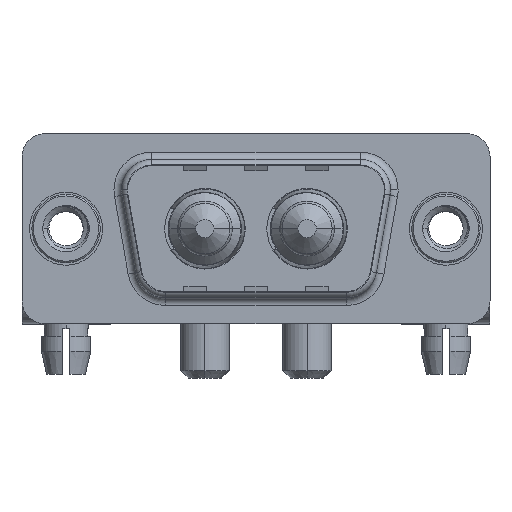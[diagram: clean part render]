
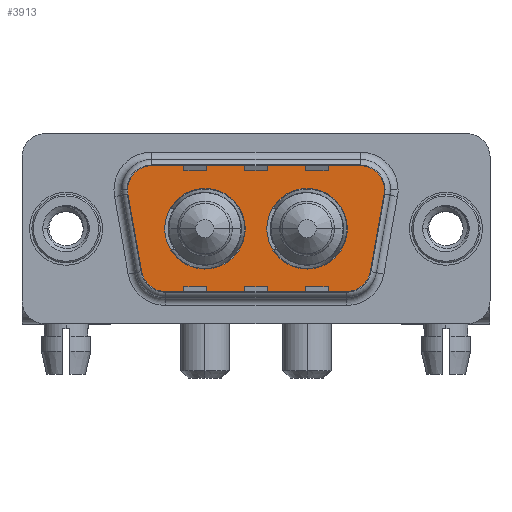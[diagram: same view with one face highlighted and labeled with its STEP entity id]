
A CAD part, top view. The second image highlights one B-rep face of the part: STEP entity #3913.
In plain terms, the highlighted planar face has unit normal (0, 0, 1).
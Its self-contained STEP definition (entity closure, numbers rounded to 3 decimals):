
#219 = ORIENTED_EDGE ( 'NONE', *, *, #4548, .T. ) ;
#256 = DIRECTION ( 'NONE',  ( -1., 0., 0. ) ) ;
#280 = CIRCLE ( 'NONE', #12714, 2.65 ) ;
#438 = VERTEX_POINT ( 'NONE', #11840 ) ;
#508 = VERTEX_POINT ( 'NONE', #8489 ) ;
#543 = CARTESIAN_POINT ( 'NONE',  ( 9.14, 0., 0. ) ) ;
#620 = AXIS2_PLACEMENT_3D ( 'NONE', #3584, #2506, #8239 ) ;
#798 = ORIENTED_EDGE ( 'NONE', *, *, #2090, .T. ) ;
#818 = EDGE_CURVE ( 'NONE', #6148, #5850, #7946, .T. ) ;
#905 = CARTESIAN_POINT ( 'NONE',  ( 4.489, -3.247, 0. ) ) ;
#919 = DIRECTION ( 'NONE',  ( 0., 0., 1. ) ) ;
#965 = CARTESIAN_POINT ( 'NONE',  ( 6.459, -4.9, 0. ) ) ;
#978 = EDGE_CURVE ( 'NONE', #4302, #438, #5430, .T. ) ;
#1011 = ORIENTED_EDGE ( 'NONE', *, *, #11360, .T. ) ;
#1084 = ORIENTED_EDGE ( 'NONE', *, *, #3416, .F. ) ;
#1127 = DIRECTION ( 'NONE',  ( 0., 0., 1. ) ) ;
#1158 = ORIENTED_EDGE ( 'NONE', *, *, #5422, .T. ) ;
#1280 = VECTOR ( 'NONE', #6122, 1000. ) ;
#1471 = ORIENTED_EDGE ( 'NONE', *, *, #11089, .F. ) ;
#1512 = DIRECTION ( 'NONE',  ( -1., 0., 0. ) ) ;
#1621 = CARTESIAN_POINT ( 'NONE',  ( 21.564, 2.9, 0. ) ) ;
#1681 = VERTEX_POINT ( 'NONE', #15098 ) ;
#2090 = EDGE_CURVE ( 'NONE', #1681, #9405, #5694, .T. ) ;
#2286 = AXIS2_PLACEMENT_3D ( 'NONE', #11740, #12900, #14204 ) ;
#2357 = VERTEX_POINT ( 'NONE', #6138 ) ;
#2362 = DIRECTION ( 'NONE',  ( 1., 0., 0. ) ) ;
#2506 = DIRECTION ( 'NONE',  ( 0., 0., 1. ) ) ;
#2527 = AXIS2_PLACEMENT_3D ( 'NONE', #4355, #4288, #8854 ) ;
#2708 = EDGE_CURVE ( 'NONE', #3065, #6148, #3999, .T. ) ;
#3010 = CIRCLE ( 'NONE', #2527, 2. ) ;
#3065 = VERTEX_POINT ( 'NONE', #10434 ) ;
#3349 = ORIENTED_EDGE ( 'NONE', *, *, #2708, .T. ) ;
#3353 = DIRECTION ( 'NONE',  ( 0.174, -0.985, 0. ) ) ;
#3416 = EDGE_CURVE ( 'NONE', #10693, #4105, #11099, .T. ) ;
#3494 = DIRECTION ( 'NONE',  ( -1., 0., 0. ) ) ;
#3502 = DIRECTION ( 'NONE',  ( 0., 0., 1. ) ) ;
#3505 = EDGE_CURVE ( 'NONE', #508, #3065, #12966, .T. ) ;
#3518 = AXIS2_PLACEMENT_3D ( 'NONE', #5768, #14240, #256 ) ;
#3584 = CARTESIAN_POINT ( 'NONE',  ( 9.14, 0., 0. ) ) ;
#3783 = AXIS2_PLACEMENT_3D ( 'NONE', #9064, #11437, #12652 ) ;
#3913 = ADVANCED_FACE ( 'NONE', ( #11501, #7924, #6779 ), #11579, .T. ) ;
#3999 = CIRCLE ( 'NONE', #2286, 2. ) ;
#4105 = VERTEX_POINT ( 'NONE', #12807 ) ;
#4218 = ORIENTED_EDGE ( 'NONE', *, *, #978, .F. ) ;
#4288 = DIRECTION ( 'NONE',  ( 0., 0., 1. ) ) ;
#4302 = VERTEX_POINT ( 'NONE', #8522 ) ;
#4355 = CARTESIAN_POINT ( 'NONE',  ( 18.541, -2.9, 0. ) ) ;
#4548 = EDGE_CURVE ( 'NONE', #13067, #508, #13030, .T. ) ;
#4737 = CARTESIAN_POINT ( 'NONE',  ( 5.436, 4.9, 0. ) ) ;
#4970 = DIRECTION ( 'NONE',  ( 1., 0., 0. ) ) ;
#5217 = LINE ( 'NONE', #9941, #1280 ) ;
#5422 = EDGE_CURVE ( 'NONE', #5850, #1681, #10359, .T. ) ;
#5430 = CIRCLE ( 'NONE', #14442, 2.65 ) ;
#5577 = CARTESIAN_POINT ( 'NONE',  ( 19.564, 2.9, 0. ) ) ;
#5694 = LINE ( 'NONE', #965, #8126 ) ;
#5768 = CARTESIAN_POINT ( 'NONE',  ( 19.564, 2.9, 0. ) ) ;
#5775 = CARTESIAN_POINT ( 'NONE',  ( 3.466, 2.553, 0. ) ) ;
#5850 = VERTEX_POINT ( 'NONE', #905 ) ;
#6122 = DIRECTION ( 'NONE',  ( 0.174, 0.985, 0. ) ) ;
#6138 = CARTESIAN_POINT ( 'NONE',  ( 21.534, 2.553, 0. ) ) ;
#6148 = VERTEX_POINT ( 'NONE', #5775 ) ;
#6239 = CIRCLE ( 'NONE', #12806, 2. ) ;
#6385 = AXIS2_PLACEMENT_3D ( 'NONE', #543, #8714, #4970 ) ;
#6779 = FACE_OUTER_BOUND ( 'NONE', #10398, .T. ) ;
#6901 = CARTESIAN_POINT ( 'NONE',  ( 20.511, -3.247, 0. ) ) ;
#7263 = VERTEX_POINT ( 'NONE', #6901 ) ;
#7321 = CARTESIAN_POINT ( 'NONE',  ( 15.86, 0., 0. ) ) ;
#7867 = CARTESIAN_POINT ( 'NONE',  ( 18.541, -4.9, 0. ) ) ;
#7924 = FACE_BOUND ( 'NONE', #9771, .T. ) ;
#7946 = LINE ( 'NONE', #8953, #8824 ) ;
#8126 = VECTOR ( 'NONE', #13867, 1000. ) ;
#8239 = DIRECTION ( 'NONE',  ( 1., 0., 0. ) ) ;
#8489 = CARTESIAN_POINT ( 'NONE',  ( 19.564, 4.9, 0. ) ) ;
#8522 = CARTESIAN_POINT ( 'NONE',  ( 13.21, 0., 0. ) ) ;
#8529 = DIRECTION ( 'NONE',  ( 1., 0., 0. ) ) ;
#8714 = DIRECTION ( 'NONE',  ( 0., 0., 1. ) ) ;
#8824 = VECTOR ( 'NONE', #3353, 1000. ) ;
#8844 = ORIENTED_EDGE ( 'NONE', *, *, #11159, .F. ) ;
#8854 = DIRECTION ( 'NONE',  ( 1., 0., 0. ) ) ;
#8953 = CARTESIAN_POINT ( 'NONE',  ( 3.466, 2.553, 0. ) ) ;
#9000 = CARTESIAN_POINT ( 'NONE',  ( 18.541, -2.9, 0. ) ) ;
#9013 = ORIENTED_EDGE ( 'NONE', *, *, #3505, .T. ) ;
#9064 = CARTESIAN_POINT ( 'NONE',  ( 6.459, -2.9, 0. ) ) ;
#9405 = VERTEX_POINT ( 'NONE', #7867 ) ;
#9673 = DIRECTION ( 'NONE',  ( 0., 0., 1. ) ) ;
#9771 = EDGE_LOOP ( 'NONE', ( #8844, #1084 ) ) ;
#9941 = CARTESIAN_POINT ( 'NONE',  ( 21.534, 2.553, 0. ) ) ;
#10254 = EDGE_CURVE ( 'NONE', #7263, #2357, #5217, .T. ) ;
#10359 = CIRCLE ( 'NONE', #3783, 2. ) ;
#10398 = EDGE_LOOP ( 'NONE', ( #1011, #12518, #14251, #219, #9013, #3349, #13445, #1158, #798 ) ) ;
#10434 = CARTESIAN_POINT ( 'NONE',  ( 5.436, 4.9, 0. ) ) ;
#10693 = VERTEX_POINT ( 'NONE', #12137 ) ;
#10813 = CARTESIAN_POINT ( 'NONE',  ( 15.86, 0., 0. ) ) ;
#11089 = EDGE_CURVE ( 'NONE', #438, #4302, #280, .T. ) ;
#11099 = CIRCLE ( 'NONE', #620, 2.65 ) ;
#11159 = EDGE_CURVE ( 'NONE', #4105, #10693, #13213, .T. ) ;
#11360 = EDGE_CURVE ( 'NONE', #9405, #7263, #3010, .T. ) ;
#11395 = EDGE_LOOP ( 'NONE', ( #1471, #4218 ) ) ;
#11436 = DIRECTION ( 'NONE',  ( 1., 0., 0. ) ) ;
#11437 = DIRECTION ( 'NONE',  ( 0., 0., 1. ) ) ;
#11501 = FACE_BOUND ( 'NONE', #11395, .T. ) ;
#11579 = PLANE ( 'NONE',  #14972 ) ;
#11740 = CARTESIAN_POINT ( 'NONE',  ( 5.436, 2.9, 0. ) ) ;
#11840 = CARTESIAN_POINT ( 'NONE',  ( 18.51, 0., 0. ) ) ;
#12137 = CARTESIAN_POINT ( 'NONE',  ( 6.49, 0., 0. ) ) ;
#12518 = ORIENTED_EDGE ( 'NONE', *, *, #10254, .T. ) ;
#12652 = DIRECTION ( 'NONE',  ( -1., 0., 0. ) ) ;
#12714 = AXIS2_PLACEMENT_3D ( 'NONE', #10813, #9673, #8529 ) ;
#12806 = AXIS2_PLACEMENT_3D ( 'NONE', #5577, #919, #3494 ) ;
#12807 = CARTESIAN_POINT ( 'NONE',  ( 11.79, 0., 0. ) ) ;
#12900 = DIRECTION ( 'NONE',  ( 0., 0., 1. ) ) ;
#12966 = LINE ( 'NONE', #4737, #14229 ) ;
#13030 = CIRCLE ( 'NONE', #3518, 2. ) ;
#13067 = VERTEX_POINT ( 'NONE', #1621 ) ;
#13213 = CIRCLE ( 'NONE', #6385, 2.65 ) ;
#13445 = ORIENTED_EDGE ( 'NONE', *, *, #818, .T. ) ;
#13867 = DIRECTION ( 'NONE',  ( 1., 0., 0. ) ) ;
#14204 = DIRECTION ( 'NONE',  ( 1., 0., 0. ) ) ;
#14229 = VECTOR ( 'NONE', #1512, 1000. ) ;
#14240 = DIRECTION ( 'NONE',  ( 0., 0., 1. ) ) ;
#14251 = ORIENTED_EDGE ( 'NONE', *, *, #14882, .T. ) ;
#14442 = AXIS2_PLACEMENT_3D ( 'NONE', #7321, #3502, #2362 ) ;
#14882 = EDGE_CURVE ( 'NONE', #2357, #13067, #6239, .T. ) ;
#14972 = AXIS2_PLACEMENT_3D ( 'NONE', #9000, #1127, #11436 ) ;
#15098 = CARTESIAN_POINT ( 'NONE',  ( 6.459, -4.9, 0. ) ) ;
